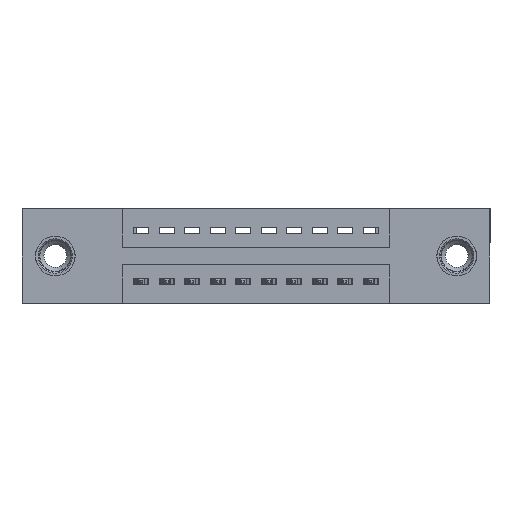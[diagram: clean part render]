
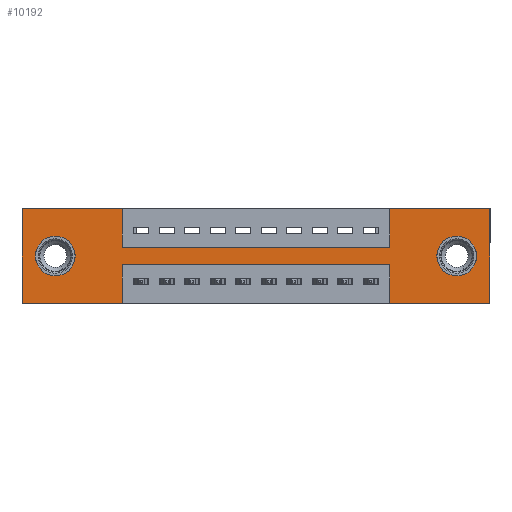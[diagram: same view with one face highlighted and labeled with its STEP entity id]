
A CAD part, front view. The second image highlights one B-rep face of the part: STEP entity #10192.
In plain terms, the highlighted planar face has unit normal (0, -1, 0).
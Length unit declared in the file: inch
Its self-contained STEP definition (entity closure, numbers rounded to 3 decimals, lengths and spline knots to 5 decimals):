
#11 = PLANE ( 'NONE',  #1651 ) ;
#182 = EDGE_CURVE ( 'NONE', #8918, #5017, #694, .T. ) ;
#271 = VECTOR ( 'NONE', #7377, 39.37008 ) ;
#322 = VERTEX_POINT ( 'NONE', #9477 ) ;
#586 = FACE_BOUND ( 'NONE', #13917, .T. ) ;
#694 = LINE ( 'NONE', #8917, #4730 ) ;
#1094 = LINE ( 'NONE', #4918, #2320 ) ;
#1145 = EDGE_LOOP ( 'NONE', ( #1407, #10523 ) ) ;
#1314 = LINE ( 'NONE', #10026, #2736 ) ;
#1317 = DIRECTION ( 'NONE',  ( 0., 0., 1. ) ) ;
#1407 = ORIENTED_EDGE ( 'NONE', *, *, #10214, .T. ) ;
#1592 = CARTESIAN_POINT ( 'NONE',  ( 1.705, 0., -0.107 ) ) ;
#1651 = AXIS2_PLACEMENT_3D ( 'NONE', #7871, #15284, #10203 ) ;
#1782 = VERTEX_POINT ( 'NONE', #16484 ) ;
#1808 = CARTESIAN_POINT ( 'NONE',  ( 0.3925, 0., -0.37 ) ) ;
#1877 = CARTESIAN_POINT ( 'NONE',  ( 0., 0., 0. ) ) ;
#1969 = ORIENTED_EDGE ( 'NONE', *, *, #14109, .F. ) ;
#2172 = EDGE_CURVE ( 'NONE', #1782, #6491, #8724, .T. ) ;
#2320 = VECTOR ( 'NONE', #4710, 39.37008 ) ;
#2542 = CARTESIAN_POINT ( 'NONE',  ( 1.835, 0., 0. ) ) ;
#2736 = VECTOR ( 'NONE', #13997, 39.37008 ) ;
#2742 = DIRECTION ( 'NONE',  ( 0., 0., 1. ) ) ;
#2791 = CARTESIAN_POINT ( 'NONE',  ( 1.705, 0., -0.185 ) ) ;
#3102 = DIRECTION ( 'NONE',  ( -1., 0., 0. ) ) ;
#3414 = VERTEX_POINT ( 'NONE', #8029 ) ;
#3426 = CARTESIAN_POINT ( 'NONE',  ( 1.705, 0., -0.185 ) ) ;
#3505 = CIRCLE ( 'NONE', #6617, 0.078 ) ;
#3922 = LINE ( 'NONE', #7197, #11378 ) ;
#4000 = CIRCLE ( 'NONE', #16565, 0.078 ) ;
#4027 = CARTESIAN_POINT ( 'NONE',  ( 0.13, 0., -0.185 ) ) ;
#4034 = ORIENTED_EDGE ( 'NONE', *, *, #11856, .T. ) ;
#4710 = DIRECTION ( 'NONE',  ( 1., 0., 0. ) ) ;
#4730 = VECTOR ( 'NONE', #13796, 39.37008 ) ;
#4755 = DIRECTION ( 'NONE',  ( 0., 0., 1. ) ) ;
#4867 = DIRECTION ( 'NONE',  ( 0., 0., -1. ) ) ;
#4918 = CARTESIAN_POINT ( 'NONE',  ( 0.3925, 0., -0.15 ) ) ;
#5017 = VERTEX_POINT ( 'NONE', #10801 ) ;
#5105 = DIRECTION ( 'NONE',  ( 0., 1., 0. ) ) ;
#5424 = CARTESIAN_POINT ( 'NONE',  ( 1.705, 0., -0.263 ) ) ;
#5588 = LINE ( 'NONE', #6640, #10574 ) ;
#5739 = DIRECTION ( 'NONE',  ( -1., 0., 0. ) ) ;
#5778 = VERTEX_POINT ( 'NONE', #5424 ) ;
#5861 = FACE_OUTER_BOUND ( 'NONE', #15035, .T. ) ;
#5862 = EDGE_CURVE ( 'NONE', #8973, #13698, #13142, .T. ) ;
#6020 = VECTOR ( 'NONE', #13478, 39.37008 ) ;
#6089 = CARTESIAN_POINT ( 'NONE',  ( 0.3925, 0., -0.22 ) ) ;
#6137 = AXIS2_PLACEMENT_3D ( 'NONE', #2791, #6687, #7982 ) ;
#6410 = ORIENTED_EDGE ( 'NONE', *, *, #9315, .F. ) ;
#6465 = LINE ( 'NONE', #1808, #13055 ) ;
#6491 = VERTEX_POINT ( 'NONE', #13483 ) ;
#6579 = CIRCLE ( 'NONE', #6137, 0.078 ) ;
#6617 = AXIS2_PLACEMENT_3D ( 'NONE', #3426, #12342, #4867 ) ;
#6640 = CARTESIAN_POINT ( 'NONE',  ( 0., 0., 0. ) ) ;
#6687 = DIRECTION ( 'NONE',  ( 0., 1., 0. ) ) ;
#6809 = CARTESIAN_POINT ( 'NONE',  ( 0.3925, 0., 0. ) ) ;
#6986 = ORIENTED_EDGE ( 'NONE', *, *, #12385, .F. ) ;
#7036 = EDGE_CURVE ( 'NONE', #15810, #5778, #3505, .T. ) ;
#7197 = CARTESIAN_POINT ( 'NONE',  ( 0., 0., -0.37 ) ) ;
#7377 = DIRECTION ( 'NONE',  ( 0., 0., -1. ) ) ;
#7422 = CARTESIAN_POINT ( 'NONE',  ( 0.13, 0., -0.263 ) ) ;
#7450 = ORIENTED_EDGE ( 'NONE', *, *, #13800, .F. ) ;
#7497 = VERTEX_POINT ( 'NONE', #8296 ) ;
#7871 = CARTESIAN_POINT ( 'NONE',  ( 0., 0., -0.37 ) ) ;
#7922 = ORIENTED_EDGE ( 'NONE', *, *, #2172, .F. ) ;
#7982 = DIRECTION ( 'NONE',  ( 0., 0., -1. ) ) ;
#8029 = CARTESIAN_POINT ( 'NONE',  ( 0., 0., -0.37 ) ) ;
#8052 = FACE_BOUND ( 'NONE', #1145, .T. ) ;
#8114 = EDGE_CURVE ( 'NONE', #11939, #12240, #14295, .T. ) ;
#8174 = ORIENTED_EDGE ( 'NONE', *, *, #11710, .F. ) ;
#8296 = CARTESIAN_POINT ( 'NONE',  ( 0., 0., 0. ) ) ;
#8355 = LINE ( 'NONE', #10014, #16136 ) ;
#8489 = ORIENTED_EDGE ( 'NONE', *, *, #5862, .F. ) ;
#8724 = LINE ( 'NONE', #14988, #14122 ) ;
#8917 = CARTESIAN_POINT ( 'NONE',  ( 1.835, 0., 0. ) ) ;
#8918 = VERTEX_POINT ( 'NONE', #2542 ) ;
#8958 = VECTOR ( 'NONE', #9361, 39.37008 ) ;
#8973 = VERTEX_POINT ( 'NONE', #11887 ) ;
#9131 = ORIENTED_EDGE ( 'NONE', *, *, #15549, .F. ) ;
#9145 = LINE ( 'NONE', #1877, #8958 ) ;
#9298 = VERTEX_POINT ( 'NONE', #15701 ) ;
#9315 = EDGE_CURVE ( 'NONE', #13698, #9927, #6465, .T. ) ;
#9361 = DIRECTION ( 'NONE',  ( 0., 0., 1. ) ) ;
#9477 = CARTESIAN_POINT ( 'NONE',  ( 0.3925, 0., -0.15 ) ) ;
#9927 = VERTEX_POINT ( 'NONE', #15854 ) ;
#10014 = CARTESIAN_POINT ( 'NONE',  ( 1.4425, 0., -0.37 ) ) ;
#10026 = CARTESIAN_POINT ( 'NONE',  ( 0., 0., -0.37 ) ) ;
#10192 = ADVANCED_FACE ( 'NONE', ( #586, #8052, #5861 ), #11, .T. ) ;
#10203 = DIRECTION ( 'NONE',  ( 0., 0., -1. ) ) ;
#10214 = EDGE_CURVE ( 'NONE', #12240, #11939, #4000, .T. ) ;
#10258 = CARTESIAN_POINT ( 'NONE',  ( 0.13, 0., -0.185 ) ) ;
#10363 = DIRECTION ( 'NONE',  ( 1., 0., 0. ) ) ;
#10433 = ORIENTED_EDGE ( 'NONE', *, *, #182, .F. ) ;
#10523 = ORIENTED_EDGE ( 'NONE', *, *, #8114, .T. ) ;
#10574 = VECTOR ( 'NONE', #10363, 39.37008 ) ;
#10588 = LINE ( 'NONE', #15857, #6020 ) ;
#10624 = DIRECTION ( 'NONE',  ( 0., 0., -1. ) ) ;
#10801 = CARTESIAN_POINT ( 'NONE',  ( 1.835, 0., -0.37 ) ) ;
#11222 = CARTESIAN_POINT ( 'NONE',  ( 0.3925, 0., 0. ) ) ;
#11261 = EDGE_CURVE ( 'NONE', #7497, #15869, #10588, .T. ) ;
#11378 = VECTOR ( 'NONE', #5739, 39.37008 ) ;
#11710 = EDGE_CURVE ( 'NONE', #6491, #8918, #5588, .T. ) ;
#11856 = EDGE_CURVE ( 'NONE', #5778, #15810, #6579, .T. ) ;
#11880 = EDGE_CURVE ( 'NONE', #322, #1782, #1094, .T. ) ;
#11887 = CARTESIAN_POINT ( 'NONE',  ( 1.4425, 0., -0.22 ) ) ;
#11939 = VERTEX_POINT ( 'NONE', #7422 ) ;
#12128 = ORIENTED_EDGE ( 'NONE', *, *, #16117, .F. ) ;
#12240 = VERTEX_POINT ( 'NONE', #14398 ) ;
#12342 = DIRECTION ( 'NONE',  ( 0., 1., 0. ) ) ;
#12385 = EDGE_CURVE ( 'NONE', #3414, #7497, #9145, .T. ) ;
#13055 = VECTOR ( 'NONE', #10624, 39.37008 ) ;
#13142 = LINE ( 'NONE', #13305, #15134 ) ;
#13305 = CARTESIAN_POINT ( 'NONE',  ( 0.3925, 0., -0.22 ) ) ;
#13478 = DIRECTION ( 'NONE',  ( 1., 0., 0. ) ) ;
#13483 = CARTESIAN_POINT ( 'NONE',  ( 1.4425, 0., 0. ) ) ;
#13551 = LINE ( 'NONE', #11222, #271 ) ;
#13698 = VERTEX_POINT ( 'NONE', #6089 ) ;
#13796 = DIRECTION ( 'NONE',  ( 0., 0., -1. ) ) ;
#13800 = EDGE_CURVE ( 'NONE', #9927, #3414, #1314, .T. ) ;
#13917 = EDGE_LOOP ( 'NONE', ( #16202, #4034 ) ) ;
#13968 = ORIENTED_EDGE ( 'NONE', *, *, #11261, .F. ) ;
#13997 = DIRECTION ( 'NONE',  ( -1., 0., 0. ) ) ;
#14109 = EDGE_CURVE ( 'NONE', #5017, #9298, #3922, .T. ) ;
#14122 = VECTOR ( 'NONE', #16265, 39.37008 ) ;
#14191 = DIRECTION ( 'NONE',  ( 0., 1., 0. ) ) ;
#14295 = CIRCLE ( 'NONE', #15380, 0.078 ) ;
#14398 = CARTESIAN_POINT ( 'NONE',  ( 0.13, 0., -0.107 ) ) ;
#14530 = ORIENTED_EDGE ( 'NONE', *, *, #11880, .F. ) ;
#14988 = CARTESIAN_POINT ( 'NONE',  ( 1.4425, 0., 0. ) ) ;
#15035 = EDGE_LOOP ( 'NONE', ( #6410, #8489, #12128, #1969, #10433, #8174, #7922, #14530, #9131, #13968, #6986, #7450 ) ) ;
#15134 = VECTOR ( 'NONE', #3102, 39.37008 ) ;
#15284 = DIRECTION ( 'NONE',  ( 0., -1., 0. ) ) ;
#15380 = AXIS2_PLACEMENT_3D ( 'NONE', #4027, #14191, #2742 ) ;
#15549 = EDGE_CURVE ( 'NONE', #15869, #322, #13551, .T. ) ;
#15701 = CARTESIAN_POINT ( 'NONE',  ( 1.4425, 0., -0.37 ) ) ;
#15810 = VERTEX_POINT ( 'NONE', #1592 ) ;
#15854 = CARTESIAN_POINT ( 'NONE',  ( 0.3925, 0., -0.37 ) ) ;
#15857 = CARTESIAN_POINT ( 'NONE',  ( 0., 0., 0. ) ) ;
#15869 = VERTEX_POINT ( 'NONE', #6809 ) ;
#16117 = EDGE_CURVE ( 'NONE', #9298, #8973, #8355, .T. ) ;
#16136 = VECTOR ( 'NONE', #4755, 39.37008 ) ;
#16202 = ORIENTED_EDGE ( 'NONE', *, *, #7036, .T. ) ;
#16265 = DIRECTION ( 'NONE',  ( 0., 0., 1. ) ) ;
#16484 = CARTESIAN_POINT ( 'NONE',  ( 1.4425, 0., -0.15 ) ) ;
#16565 = AXIS2_PLACEMENT_3D ( 'NONE', #10258, #5105, #1317 ) ;
